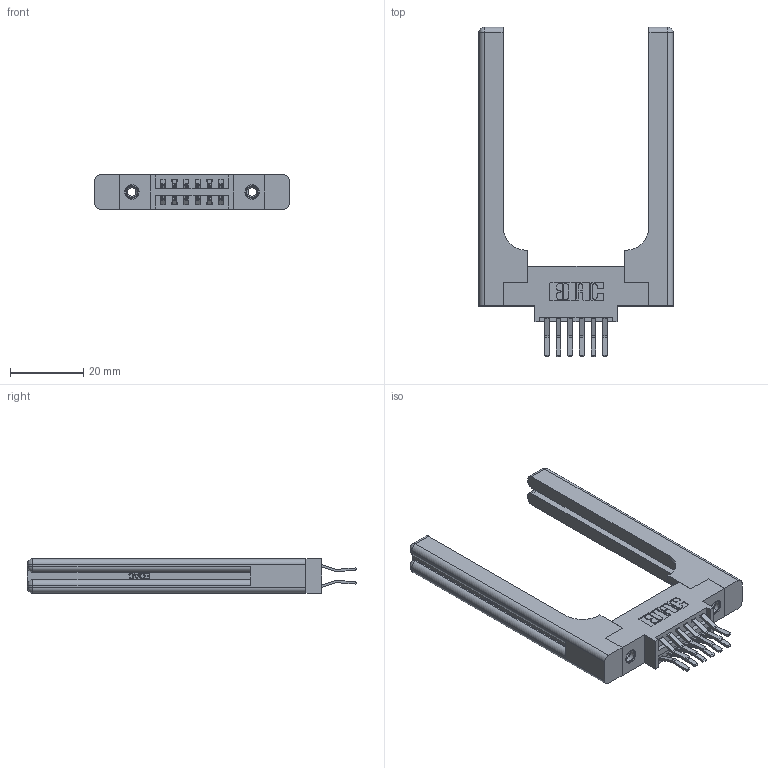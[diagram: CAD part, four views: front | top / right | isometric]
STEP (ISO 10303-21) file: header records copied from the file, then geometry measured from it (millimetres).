
FILE_DESCRIPTION (( 'STEP AP203' ), '1' );
FILE_NAME ('346-012-560-858.STEP', '2022-05-18T13:47:09', ( '' ), ( '' ), 'SwSTEP 2.0', 'SolidWorks 2020', '' );
FILE_SCHEMA (( 'CONFIG_CONTROL_DESIGN' ));
Length unit declared in the file: inch
Products named in the file (5): 345-250-001_345-250-001-102; 346 Part_0.170 Offset - 0.156 Dia-TH; 346-220-058_345-220-058; 346-012-560-858; 345-292-001_560 Tail
Assembly tree (17 placements, depth 2):
  346-012-560-858
    346 Part_0.170 Offset - 0.156 Dia-TH
    345-292-001_560 Tail  x12
    345-250-001_345-250-001-102  x2
    346-220-058_345-220-058  x2
Bounding box: 53.11 x 90.05 x 9.4 mm (x, y, z)
Volume: 12299.6 mm3; surface area: 11436.3 mm2
Topology: 17 solids, 17 shells, 1044 faces, 2975 edges, 1946 vertices
Faces by surface type: plane 662, cylinder 322, bspline 36, cone 12, sphere 8, torus 4
Entity records: 14580 total; most frequent: CARTESIAN_POINT 3467, ORIENTED_EDGE 2196, DIRECTION 2042, EDGE_CURVE 1098, LINE 846, VECTOR 846, VERTEX_POINT 722, AXIS2_PLACEMENT_3D 598
